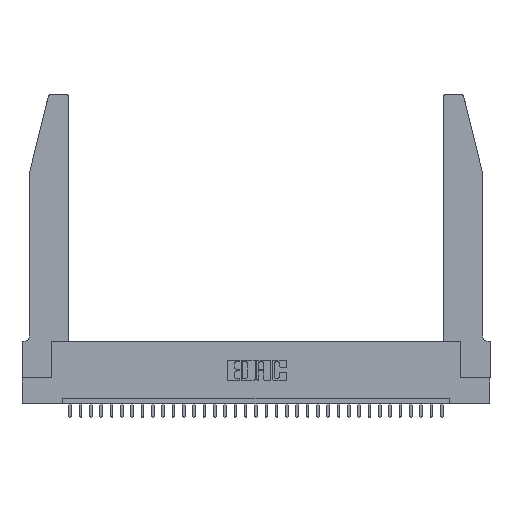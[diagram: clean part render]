
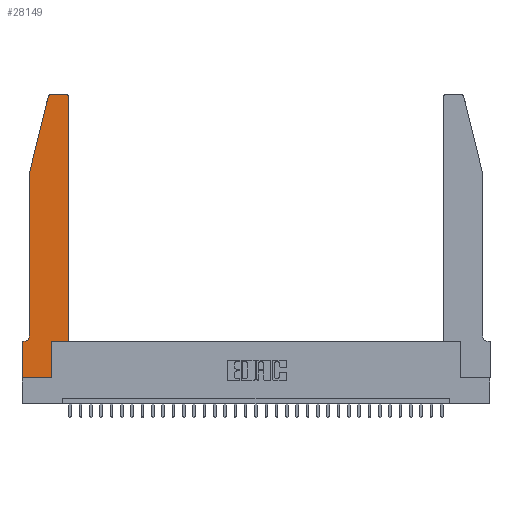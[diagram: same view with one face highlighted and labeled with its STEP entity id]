
A CAD part, top view. The second image highlights one B-rep face of the part: STEP entity #28149.
In plain terms, the highlighted planar face has unit normal (0, 0, 1).
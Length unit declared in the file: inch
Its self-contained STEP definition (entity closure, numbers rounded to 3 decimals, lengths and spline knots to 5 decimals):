
#750 = DIRECTION ( 'NONE',  ( -1., 0., 0. ) ) ;
#1191 = EDGE_CURVE ( 'NONE', #22447, #24305, #23990, .T. ) ;
#1423 = DIRECTION ( 'NONE',  ( 0., 0., 1. ) ) ;
#2136 = CARTESIAN_POINT ( 'NONE',  ( 0.284, 2.72, 0.37 ) ) ;
#2689 = EDGE_CURVE ( 'NONE', #20487, #19971, #27526, .T. ) ;
#2929 = ORIENTED_EDGE ( 'NONE', *, *, #3771, .T. ) ;
#3113 = EDGE_CURVE ( 'NONE', #12854, #15360, #9033, .T. ) ;
#3771 = EDGE_CURVE ( 'NONE', #9271, #12854, #7734, .T. ) ;
#3798 = DIRECTION ( 'NONE',  ( 0., 1., 0. ) ) ;
#4174 = VERTEX_POINT ( 'NONE', #31672 ) ;
#4252 = CARTESIAN_POINT ( 'NONE',  ( 0., 0.35, 0.37 ) ) ;
#4502 = ORIENTED_EDGE ( 'NONE', *, *, #3113, .T. ) ;
#4565 = CARTESIAN_POINT ( 'NONE',  ( 0.4205, 2.75, 0.37 ) ) ;
#5244 = DIRECTION ( 'NONE',  ( 0., 0., -1. ) ) ;
#5473 = LINE ( 'NONE', #18800, #32803 ) ;
#5691 = CARTESIAN_POINT ( 'NONE',  ( 0.0755, 0.35, 0.37 ) ) ;
#5774 = CARTESIAN_POINT ( 'NONE',  ( 0.0055, 0.35, 0.37 ) ) ;
#6121 = CARTESIAN_POINT ( 'NONE',  ( 0.0755, 0.42, 0.37 ) ) ;
#6609 = VECTOR ( 'NONE', #750, 39.37008 ) ;
#6722 = CARTESIAN_POINT ( 'NONE',  ( 0.2865, 0., 0.37 ) ) ;
#7339 = DIRECTION ( 'NONE',  ( 0., -1., 0. ) ) ;
#7341 = VECTOR ( 'NONE', #27796, 39.37008 ) ;
#7734 = LINE ( 'NONE', #30747, #7341 ) ;
#7750 = EDGE_CURVE ( 'NONE', #25483, #17029, #7841, .T. ) ;
#7841 = LINE ( 'NONE', #14453, #27513 ) ;
#8526 = CARTESIAN_POINT ( 'NONE',  ( 0.0755, 2., 0.37 ) ) ;
#8825 = EDGE_LOOP ( 'NONE', ( #27386, #28505, #20691, #14921, #15915, #12441, #12404, #10022, #20653, #2929, #4502, #17806 ) ) ;
#9033 = LINE ( 'NONE', #23175, #16249 ) ;
#9271 = VERTEX_POINT ( 'NONE', #16535 ) ;
#9307 = VECTOR ( 'NONE', #19768, 39.37008 ) ;
#9520 = VECTOR ( 'NONE', #25550, 39.37008 ) ;
#9639 = AXIS2_PLACEMENT_3D ( 'NONE', #10807, #18528, #13279 ) ;
#10022 = ORIENTED_EDGE ( 'NONE', *, *, #10118, .T. ) ;
#10118 = EDGE_CURVE ( 'NONE', #4174, #33024, #15706, .T. ) ;
#10201 = CARTESIAN_POINT ( 'NONE',  ( 0.0055, 0.42, 0.37 ) ) ;
#10807 = CARTESIAN_POINT ( 'NONE',  ( 0., 0.35, 0.37 ) ) ;
#11322 = CARTESIAN_POINT ( 'NONE',  ( 0.4205, 2.72, 0.37 ) ) ;
#11620 = EDGE_CURVE ( 'NONE', #33024, #9271, #12412, .T. ) ;
#11863 = AXIS2_PLACEMENT_3D ( 'NONE', #10201, #5244, #13227 ) ;
#12404 = ORIENTED_EDGE ( 'NONE', *, *, #19236, .T. ) ;
#12412 = LINE ( 'NONE', #13254, #32878 ) ;
#12441 = ORIENTED_EDGE ( 'NONE', *, *, #14164, .T. ) ;
#12472 = AXIS2_PLACEMENT_3D ( 'NONE', #11322, #1423, #31750 ) ;
#12628 = CARTESIAN_POINT ( 'NONE',  ( 0.0755, 2., 0.37 ) ) ;
#12763 = EDGE_CURVE ( 'NONE', #24305, #20487, #14345, .T. ) ;
#12854 = VERTEX_POINT ( 'NONE', #24792 ) ;
#13227 = DIRECTION ( 'NONE',  ( -1., 0., 0. ) ) ;
#13254 = CARTESIAN_POINT ( 'NONE',  ( 0.2865, 0.35, 0.37 ) ) ;
#13279 = DIRECTION ( 'NONE',  ( 1., 0., 0. ) ) ;
#14164 = EDGE_CURVE ( 'NONE', #19971, #31043, #27073, .T. ) ;
#14345 = LINE ( 'NONE', #12628, #20326 ) ;
#14453 = CARTESIAN_POINT ( 'NONE',  ( 0.2605, 2.75, 0.37 ) ) ;
#14637 = CARTESIAN_POINT ( 'NONE',  ( 0., 0., 0.37 ) ) ;
#14921 = ORIENTED_EDGE ( 'NONE', *, *, #12763, .T. ) ;
#14941 = AXIS2_PLACEMENT_3D ( 'NONE', #2136, #17274, #30224 ) ;
#15360 = VERTEX_POINT ( 'NONE', #29459 ) ;
#15706 = LINE ( 'NONE', #14637, #9307 ) ;
#15773 = CARTESIAN_POINT ( 'NONE',  ( 0.0755, 2., 0.37 ) ) ;
#15915 = ORIENTED_EDGE ( 'NONE', *, *, #2689, .T. ) ;
#16249 = VECTOR ( 'NONE', #28515, 39.37008 ) ;
#16535 = CARTESIAN_POINT ( 'NONE',  ( 0.2865, 0.35, 0.37 ) ) ;
#17029 = VERTEX_POINT ( 'NONE', #26729 ) ;
#17108 = DIRECTION ( 'NONE',  ( -1., 0., 0. ) ) ;
#17274 = DIRECTION ( 'NONE',  ( 0., 0., 1. ) ) ;
#17357 = FACE_OUTER_BOUND ( 'NONE', #8825, .T. ) ;
#17806 = ORIENTED_EDGE ( 'NONE', *, *, #25829, .T. ) ;
#18528 = DIRECTION ( 'NONE',  ( 0., 0., 1. ) ) ;
#18800 = CARTESIAN_POINT ( 'NONE',  ( 0., 0., 0.37 ) ) ;
#19236 = EDGE_CURVE ( 'NONE', #31043, #4174, #5473, .T. ) ;
#19768 = DIRECTION ( 'NONE',  ( 1., 0., 0. ) ) ;
#19971 = VERTEX_POINT ( 'NONE', #5774 ) ;
#20326 = VECTOR ( 'NONE', #7339, 39.37008 ) ;
#20487 = VERTEX_POINT ( 'NONE', #6121 ) ;
#20653 = ORIENTED_EDGE ( 'NONE', *, *, #11620, .T. ) ;
#20691 = ORIENTED_EDGE ( 'NONE', *, *, #1191, .T. ) ;
#20933 = CIRCLE ( 'NONE', #14941, 0.03 ) ;
#21588 = EDGE_CURVE ( 'NONE', #17029, #22447, #20933, .T. ) ;
#22447 = VERTEX_POINT ( 'NONE', #25089 ) ;
#23175 = CARTESIAN_POINT ( 'NONE',  ( 0.4505, 0.35, 0.37 ) ) ;
#23610 = PLANE ( 'NONE',  #9639 ) ;
#23747 = DIRECTION ( 'NONE',  ( 0., -1., 0. ) ) ;
#23990 = LINE ( 'NONE', #15773, #9520 ) ;
#24305 = VERTEX_POINT ( 'NONE', #8526 ) ;
#24792 = CARTESIAN_POINT ( 'NONE',  ( 0.4505, 0.35, 0.37 ) ) ;
#25089 = CARTESIAN_POINT ( 'NONE',  ( 0.25487, 2.72718, 0.37 ) ) ;
#25483 = VERTEX_POINT ( 'NONE', #4565 ) ;
#25550 = DIRECTION ( 'NONE',  ( -0.239, -0.971, 0. ) ) ;
#25829 = EDGE_CURVE ( 'NONE', #15360, #25483, #33238, .T. ) ;
#26729 = CARTESIAN_POINT ( 'NONE',  ( 0.284, 2.75, 0.37 ) ) ;
#27073 = LINE ( 'NONE', #5691, #6609 ) ;
#27386 = ORIENTED_EDGE ( 'NONE', *, *, #7750, .T. ) ;
#27513 = VECTOR ( 'NONE', #17108, 39.37008 ) ;
#27526 = CIRCLE ( 'NONE', #11863, 0.07 ) ;
#27796 = DIRECTION ( 'NONE',  ( 1., 0., 0. ) ) ;
#28149 = ADVANCED_FACE ( 'NONE', ( #17357 ), #23610, .T. ) ;
#28505 = ORIENTED_EDGE ( 'NONE', *, *, #21588, .T. ) ;
#28515 = DIRECTION ( 'NONE',  ( 0., 1., 0. ) ) ;
#29459 = CARTESIAN_POINT ( 'NONE',  ( 0.4505, 2.72, 0.37 ) ) ;
#30224 = DIRECTION ( 'NONE',  ( 1., 0., 0. ) ) ;
#30747 = CARTESIAN_POINT ( 'NONE',  ( 0.4505, 0.35, 0.37 ) ) ;
#31043 = VERTEX_POINT ( 'NONE', #4252 ) ;
#31672 = CARTESIAN_POINT ( 'NONE',  ( 0., 0., 0.37 ) ) ;
#31750 = DIRECTION ( 'NONE',  ( 1., 0., 0. ) ) ;
#32803 = VECTOR ( 'NONE', #23747, 39.37008 ) ;
#32878 = VECTOR ( 'NONE', #3798, 39.37008 ) ;
#33024 = VERTEX_POINT ( 'NONE', #6722 ) ;
#33238 = CIRCLE ( 'NONE', #12472, 0.03 ) ;
